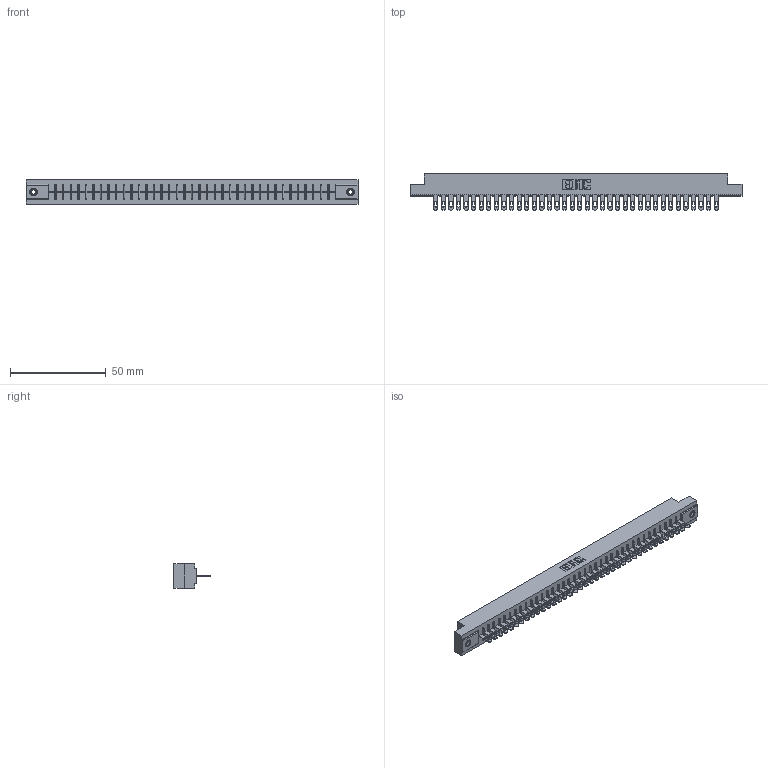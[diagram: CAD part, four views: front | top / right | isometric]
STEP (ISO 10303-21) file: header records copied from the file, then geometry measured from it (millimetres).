
FILE_DESCRIPTION (( 'STEP AP203' ), '1' );
FILE_NAME ('306-038-500-108.STEP', '2019-09-11T23:53:56', ( '' ), ( '' ), 'SwSTEP 2.0', 'SolidWorks 2016', '' );
FILE_SCHEMA (( 'CONFIG_CONTROL_DESIGN' ));
Length unit declared in the file: inch
Products named in the file (4): 306-290-001_100; 345-250-001_345-250-003-102; 306 Part_.156 Dia; 306-038-500-108
Assembly tree (41 placements, depth 2):
  306-038-500-108
    306 Part_.156 Dia
    306-290-001_100  x38
    345-250-001_345-250-003-102  x2
Bounding box: 173.58 x 18.87 x 12.7 mm (x, y, z)
Volume: 19274.9 mm3; surface area: 20436.2 mm2
Topology: 41 solids, 41 shells, 3064 faces, 8622 edges, 5536 vertices
Faces by surface type: plane 2000, cylinder 896, sphere 152, cone 12, torus 4
Entity records: 37304 total; most frequent: CARTESIAN_POINT 6244, ORIENTED_EDGE 6184, DIRECTION 6166, EDGE_CURVE 3092, VECTOR 2414, LINE 2414, VERTEX_POINT 1954, AXIS2_PLACEMENT_3D 1876
